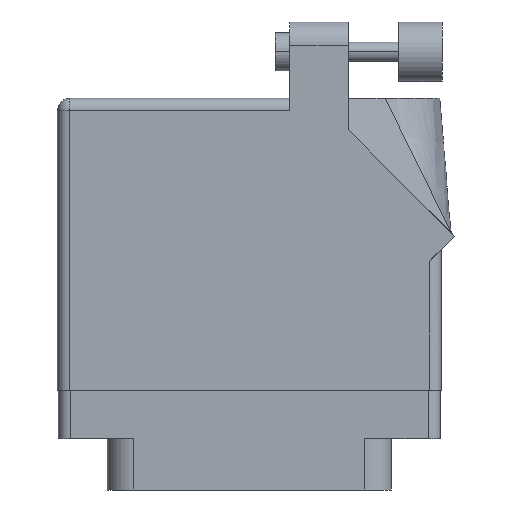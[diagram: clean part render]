
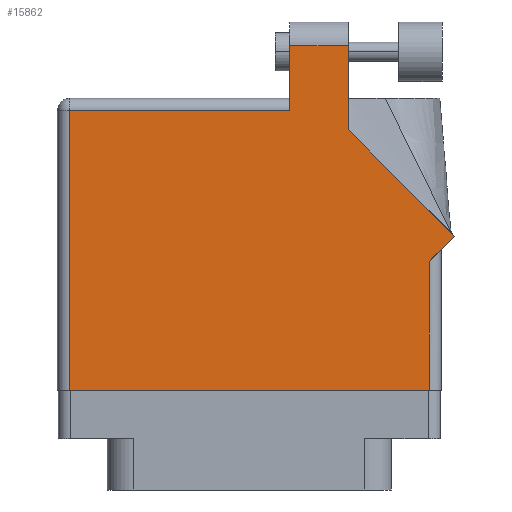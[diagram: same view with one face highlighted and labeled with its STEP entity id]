
A CAD part, front view. The second image highlights one B-rep face of the part: STEP entity #15862.
In plain terms, the highlighted face is planar.
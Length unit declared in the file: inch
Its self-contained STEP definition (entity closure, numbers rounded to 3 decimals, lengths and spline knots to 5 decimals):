
#1628 = VERTEX_POINT ( 'NONE', #5419 ) ;
#1639 = EDGE_CURVE ( 'NONE', #1628, #28501, #29695, .T. ) ;
#1929 = ORIENTED_EDGE ( 'NONE', *, *, #34915, .T. ) ;
#2210 = EDGE_CURVE ( 'NONE', #6613, #18273, #5924, .T. ) ;
#2462 = LINE ( 'NONE', #19219, #25695 ) ;
#2596 = VECTOR ( 'NONE', #14152, 39.37008 ) ;
#3519 = VECTOR ( 'NONE', #5537, 39.37008 ) ;
#5161 = VECTOR ( 'NONE', #16562, 39.37008 ) ;
#5419 = CARTESIAN_POINT ( 'NONE',  ( 0.212, 1.368, 0.455 ) ) ;
#5525 = CARTESIAN_POINT ( 'NONE',  ( 0.943, -0.1, 0.455 ) ) ;
#5537 = DIRECTION ( 'NONE',  ( 1., 0., 0. ) ) ;
#5857 = VERTEX_POINT ( 'NONE', #22322 ) ;
#5924 = LINE ( 'NONE', #11358, #33045 ) ;
#6338 = LINE ( 'NONE', #14701, #2596 ) ;
#6613 = VERTEX_POINT ( 'NONE', #32471 ) ;
#7787 = CARTESIAN_POINT ( 'NONE',  ( -1.005, 1.368, 0.455 ) ) ;
#8320 = FACE_OUTER_BOUND ( 'NONE', #23013, .T. ) ;
#8641 = ORIENTED_EDGE ( 'NONE', *, *, #17470, .T. ) ;
#8702 = ORIENTED_EDGE ( 'NONE', *, *, #27654, .T. ) ;
#10602 = CARTESIAN_POINT ( 'NONE',  ( 0.212, 1.705, 0.455 ) ) ;
#10640 = CARTESIAN_POINT ( 'NONE',  ( 0.519, 1.26442, 0.455 ) ) ;
#11118 = LINE ( 'NONE', #33005, #5161 ) ;
#11358 = CARTESIAN_POINT ( 'NONE',  ( 1.005, 0.637, 0.455 ) ) ;
#11525 = EDGE_CURVE ( 'NONE', #33823, #6613, #24896, .T. ) ;
#12521 = DIRECTION ( 'NONE',  ( 0., 1., 0. ) ) ;
#13428 = DIRECTION ( 'NONE',  ( -1., 0., 0. ) ) ;
#13933 = VERTEX_POINT ( 'NONE', #10602 ) ;
#13993 = VECTOR ( 'NONE', #14813, 39.37008 ) ;
#14064 = ORIENTED_EDGE ( 'NONE', *, *, #2210, .T. ) ;
#14152 = DIRECTION ( 'NONE',  ( -0.707, 0.707, 0. ) ) ;
#14345 = ORIENTED_EDGE ( 'NONE', *, *, #11525, .T. ) ;
#14701 = CARTESIAN_POINT ( 'NONE',  ( 1.07571, 0.70771, 0.455 ) ) ;
#14813 = DIRECTION ( 'NONE',  ( 0., -1., 0. ) ) ;
#15862 = ADVANCED_FACE ( 'NONE', ( #8320 ), #26946, .F. ) ;
#16562 = DIRECTION ( 'NONE',  ( -1., 0., 0. ) ) ;
#16658 = CARTESIAN_POINT ( 'NONE',  ( 0.943, 0.637, 0.455 ) ) ;
#17470 = EDGE_CURVE ( 'NONE', #18273, #31227, #6338, .T. ) ;
#17685 = VECTOR ( 'NONE', #19780, 39.37008 ) ;
#18273 = VERTEX_POINT ( 'NONE', #19354 ) ;
#19219 = CARTESIAN_POINT ( 'NONE',  ( -0.943, -0.1, 0.455 ) ) ;
#19354 = CARTESIAN_POINT ( 'NONE',  ( 1.07571, 0.70771, 0.455 ) ) ;
#19780 = DIRECTION ( 'NONE',  ( 0., 1., 0. ) ) ;
#20646 = ORIENTED_EDGE ( 'NONE', *, *, #22341, .T. ) ;
#21032 = LINE ( 'NONE', #23583, #13993 ) ;
#21132 = ORIENTED_EDGE ( 'NONE', *, *, #31494, .T. ) ;
#22322 = CARTESIAN_POINT ( 'NONE',  ( -0.943, -0.1, 0.455 ) ) ;
#22341 = EDGE_CURVE ( 'NONE', #28501, #5857, #2462, .T. ) ;
#23013 = EDGE_LOOP ( 'NONE', ( #1929, #8702, #21132, #27879, #20646, #25803, #14345, #14064, #8641 ) ) ;
#23583 = CARTESIAN_POINT ( 'NONE',  ( 0.212, 1.43, 0.455 ) ) ;
#24038 = DIRECTION ( 'NONE',  ( -1., 0., 0. ) ) ;
#24873 = DIRECTION ( 'NONE',  ( 0.707, 0.707, 0. ) ) ;
#24896 = LINE ( 'NONE', #16658, #17685 ) ;
#25695 = VECTOR ( 'NONE', #30365, 39.37008 ) ;
#25803 = ORIENTED_EDGE ( 'NONE', *, *, #30116, .T. ) ;
#26573 = CARTESIAN_POINT ( 'NONE',  ( 0.519, 1.26442, 0.455 ) ) ;
#26946 = PLANE ( 'NONE',  #35009 ) ;
#27654 = EDGE_CURVE ( 'NONE', #30275, #13933, #11118, .T. ) ;
#27879 = ORIENTED_EDGE ( 'NONE', *, *, #1639, .T. ) ;
#28501 = VERTEX_POINT ( 'NONE', #28692 ) ;
#28692 = CARTESIAN_POINT ( 'NONE',  ( -0.943, 1.368, 0.455 ) ) ;
#29675 = LINE ( 'NONE', #26573, #33667 ) ;
#29695 = LINE ( 'NONE', #7787, #35354 ) ;
#30116 = EDGE_CURVE ( 'NONE', #5857, #33823, #35991, .T. ) ;
#30275 = VERTEX_POINT ( 'NONE', #31604 ) ;
#30365 = DIRECTION ( 'NONE',  ( 0., -1., 0. ) ) ;
#30885 = CARTESIAN_POINT ( 'NONE',  ( -1.005, -0.1, 0.455 ) ) ;
#31227 = VERTEX_POINT ( 'NONE', #10640 ) ;
#31494 = EDGE_CURVE ( 'NONE', #13933, #1628, #21032, .T. ) ;
#31604 = CARTESIAN_POINT ( 'NONE',  ( 0.519, 1.705, 0.455 ) ) ;
#32471 = CARTESIAN_POINT ( 'NONE',  ( 0.943, 0.575, 0.455 ) ) ;
#32601 = DIRECTION ( 'NONE',  ( 0., 0., -1. ) ) ;
#33005 = CARTESIAN_POINT ( 'NONE',  ( 0.212, 1.705, 0.455 ) ) ;
#33045 = VECTOR ( 'NONE', #24873, 39.37008 ) ;
#33667 = VECTOR ( 'NONE', #12521, 39.37008 ) ;
#33823 = VERTEX_POINT ( 'NONE', #5525 ) ;
#34915 = EDGE_CURVE ( 'NONE', #31227, #30275, #29675, .T. ) ;
#35009 = AXIS2_PLACEMENT_3D ( 'NONE', #35339, #32601, #13428 ) ;
#35339 = CARTESIAN_POINT ( 'NONE',  ( -1.005, 1.43, 0.455 ) ) ;
#35354 = VECTOR ( 'NONE', #24038, 39.37008 ) ;
#35991 = LINE ( 'NONE', #30885, #3519 ) ;
